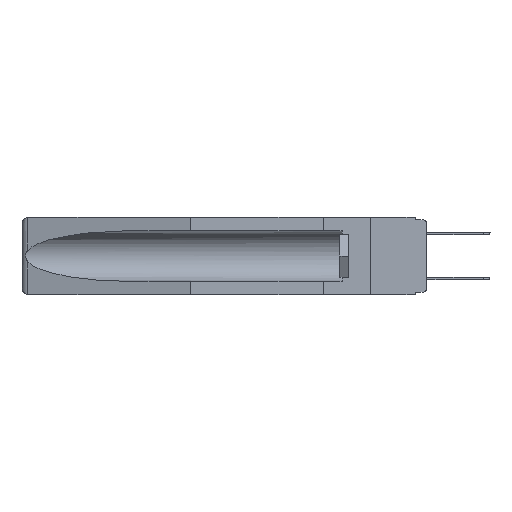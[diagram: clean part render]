
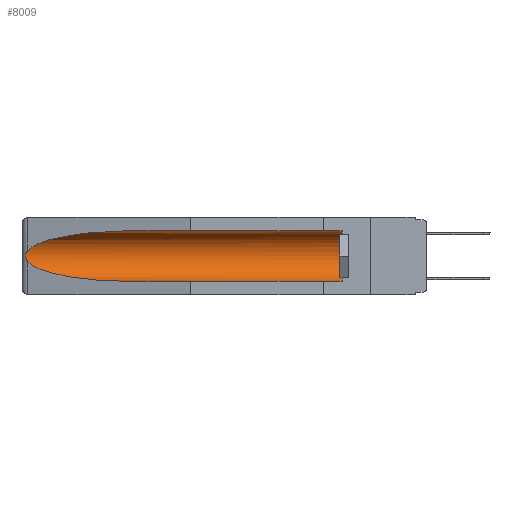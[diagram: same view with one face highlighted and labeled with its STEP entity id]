
A CAD part, left-side view. The second image highlights one B-rep face of the part: STEP entity #8009.
In plain terms, the highlighted cylindrical face has radius 2.857 mm (diameter 5.715 mm), a partial arc.
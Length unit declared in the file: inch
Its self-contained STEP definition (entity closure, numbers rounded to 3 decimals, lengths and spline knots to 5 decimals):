
#921 = CARTESIAN_POINT ( 'NONE',  ( 0.26654, 1.53092, -0.15636 ) ) ;
#1073 = CARTESIAN_POINT ( 'NONE',  ( 0.2673, 1.5327, -0.16383 ) ) ;
#2329 =( BOUNDED_CURVE ( )  B_SPLINE_CURVE ( 3, ( #11406, #5093, #13542, #17701 ),
 .UNSPECIFIED., .F., .T. ) 
 B_SPLINE_CURVE_WITH_KNOTS ( ( 4, 4 ),
 ( 4.71239, 6.08839 ),
 .UNSPECIFIED. ) 
 CURVE ( )  GEOMETRIC_REPRESENTATION_ITEM ( )  RATIONAL_B_SPLINE_CURVE ( ( 1., 0.848, 0.848, 1. ) ) 
 REPRESENTATION_ITEM ( '' )  );
#2622 = DIRECTION ( 'NONE',  ( 0., 1., 0. ) ) ;
#2668 = CARTESIAN_POINT ( 'NONE',  ( 0.2673, 1.53269, -0.17917 ) ) ;
#2696 = EDGE_CURVE ( 'NONE', #8767, #15626, #2329, .T. ) ;
#2737 = CARTESIAN_POINT ( 'NONE',  ( 0.21114, 1.30732, -0.284 ) ) ;
#3047 = CARTESIAN_POINT ( 'NONE',  ( 0.155, -0.30754, -0.1715 ) ) ;
#3201 = DIRECTION ( 'NONE',  ( 0., 0., 1. ) ) ;
#4054 = EDGE_CURVE ( 'NONE', #14514, #8767, #19173, .T. ) ;
#4633 = CARTESIAN_POINT ( 'NONE',  ( 0.155, 0.126, -0.284 ) ) ;
#5093 = CARTESIAN_POINT ( 'NONE',  ( 0.21114, 1.30732, -0.059 ) ) ;
#5690 = ORIENTED_EDGE ( 'NONE', *, *, #4054, .T. ) ;
#5698 = DIRECTION ( 'NONE',  ( 0., 1., 0. ) ) ;
#6895 = FACE_OUTER_BOUND ( 'NONE', #27007, .T. ) ;
#7523 = CARTESIAN_POINT ( 'NONE',  ( 0.26597, 1.52961, -0.15275 ) ) ;
#8009 = ADVANCED_FACE ( 'NONE', ( #6895 ), #18215, .F. ) ;
#8105 = CARTESIAN_POINT ( 'NONE',  ( 0.155, 0.126, -0.1715 ) ) ;
#8413 = DIRECTION ( 'NONE',  ( 0., 1., 0. ) ) ;
#8643 = ORIENTED_EDGE ( 'NONE', *, *, #19508, .T. ) ;
#8767 = VERTEX_POINT ( 'NONE', #11084 ) ;
#9218 = CARTESIAN_POINT ( 'NONE',  ( 0.26537, 1.52718, -0.14972 ) ) ;
#9391 = CARTESIAN_POINT ( 'NONE',  ( 0.26597, 1.5296, -0.19026 ) ) ;
#9676 = CARTESIAN_POINT ( 'NONE',  ( 0.26655, 1.53094, -0.18657 ) ) ;
#9796 = EDGE_CURVE ( 'NONE', #26256, #22199, #26838, .T. ) ;
#9817 = CARTESIAN_POINT ( 'NONE',  ( 0.2675, 1.53308, -0.16763 ) ) ;
#11084 = CARTESIAN_POINT ( 'NONE',  ( 0.155, 1.07973, -0.059 ) ) ;
#11406 = CARTESIAN_POINT ( 'NONE',  ( 0.155, 1.07973, -0.059 ) ) ;
#11754 = CARTESIAN_POINT ( 'NONE',  ( 0.155, 1.07973, -0.284 ) ) ;
#12706 = CARTESIAN_POINT ( 'NONE',  ( 0.155, -0.30754, -0.284 ) ) ;
#12791 = VECTOR ( 'NONE', #5698, 39.37008 ) ;
#13542 = CARTESIAN_POINT ( 'NONE',  ( 0.25451, 1.48313, -0.09465 ) ) ;
#14514 = VERTEX_POINT ( 'NONE', #14777 ) ;
#14643 = B_SPLINE_CURVE_WITH_KNOTS ( 'NONE', 3,
 ( #27010, #7523, #921, #1073, #9817, #25015, #2668, #9676, #9391, #24875 ),
 .UNSPECIFIED., .F., .F.,
 ( 4, 2, 2, 2, 4 ),
 ( 0., 0.00029, 0.00058, 0.00087, 0.00117 ),
 .UNSPECIFIED. ) ;
#14777 = CARTESIAN_POINT ( 'NONE',  ( 0.155, 0.126, -0.059 ) ) ;
#15218 = ORIENTED_EDGE ( 'NONE', *, *, #18302, .F. ) ;
#15626 = VERTEX_POINT ( 'NONE', #9218 ) ;
#15752 = CARTESIAN_POINT ( 'NONE',  ( 0.25451, 1.48313, -0.24835 ) ) ;
#15801 = ORIENTED_EDGE ( 'NONE', *, *, #9796, .T. ) ;
#16857 = DIRECTION ( 'NONE',  ( 0., -1., 0. ) ) ;
#17701 = CARTESIAN_POINT ( 'NONE',  ( 0.26537, 1.52718, -0.14972 ) ) ;
#18051 = CARTESIAN_POINT ( 'NONE',  ( 0.155, 1.07973, -0.284 ) ) ;
#18215 = CYLINDRICAL_SURFACE ( 'NONE', #24211, 0.1125 ) ;
#18302 = EDGE_CURVE ( 'NONE', #18844, #22199, #28043, .T. ) ;
#18473 = VECTOR ( 'NONE', #8413, 39.37008 ) ;
#18844 = VERTEX_POINT ( 'NONE', #4633 ) ;
#19173 = LINE ( 'NONE', #25340, #12791 ) ;
#19508 = EDGE_CURVE ( 'NONE', #15626, #26256, #14643, .T. ) ;
#19652 = CIRCLE ( 'NONE', #27888, 0.1125 ) ;
#21426 = CARTESIAN_POINT ( 'NONE',  ( 0.26537, 1.52718, -0.19328 ) ) ;
#21596 = DIRECTION ( 'NONE',  ( 0., 0., 1. ) ) ;
#22199 = VERTEX_POINT ( 'NONE', #18051 ) ;
#22237 = CARTESIAN_POINT ( 'NONE',  ( 0.26537, 1.52718, -0.19328 ) ) ;
#23841 = ORIENTED_EDGE ( 'NONE', *, *, #27175, .T. ) ;
#24211 = AXIS2_PLACEMENT_3D ( 'NONE', #3047, #2622, #3201 ) ;
#24875 = CARTESIAN_POINT ( 'NONE',  ( 0.26537, 1.52718, -0.19328 ) ) ;
#25015 = CARTESIAN_POINT ( 'NONE',  ( 0.2675, 1.53308, -0.17534 ) ) ;
#25340 = CARTESIAN_POINT ( 'NONE',  ( 0.155, -0.30754, -0.059 ) ) ;
#25447 = ORIENTED_EDGE ( 'NONE', *, *, #2696, .T. ) ;
#26256 = VERTEX_POINT ( 'NONE', #21426 ) ;
#26838 =( BOUNDED_CURVE ( )  B_SPLINE_CURVE ( 3, ( #22237, #15752, #2737, #11754 ),
 .UNSPECIFIED., .F., .T. ) 
 B_SPLINE_CURVE_WITH_KNOTS ( ( 4, 4 ),
 ( 0.1948, 1.5708 ),
 .UNSPECIFIED. ) 
 CURVE ( )  GEOMETRIC_REPRESENTATION_ITEM ( )  RATIONAL_B_SPLINE_CURVE ( ( 1., 0.848, 0.848, 1. ) ) 
 REPRESENTATION_ITEM ( '' )  );
#27007 = EDGE_LOOP ( 'NONE', ( #25447, #8643, #15801, #15218, #23841, #5690 ) ) ;
#27010 = CARTESIAN_POINT ( 'NONE',  ( 0.26537, 1.52718, -0.14972 ) ) ;
#27175 = EDGE_CURVE ( 'NONE', #18844, #14514, #19652, .T. ) ;
#27888 = AXIS2_PLACEMENT_3D ( 'NONE', #8105, #16857, #21596 ) ;
#28043 = LINE ( 'NONE', #12706, #18473 ) ;
